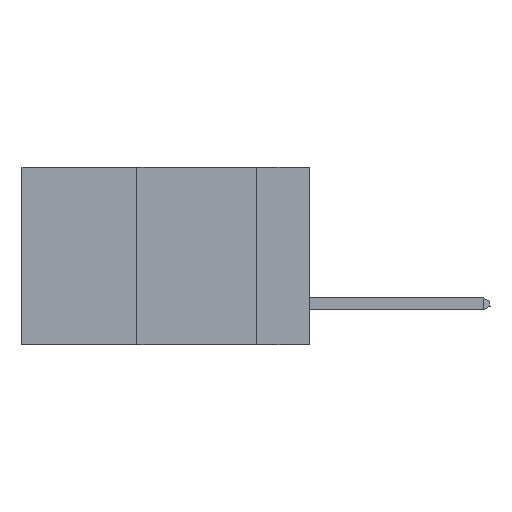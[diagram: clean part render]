
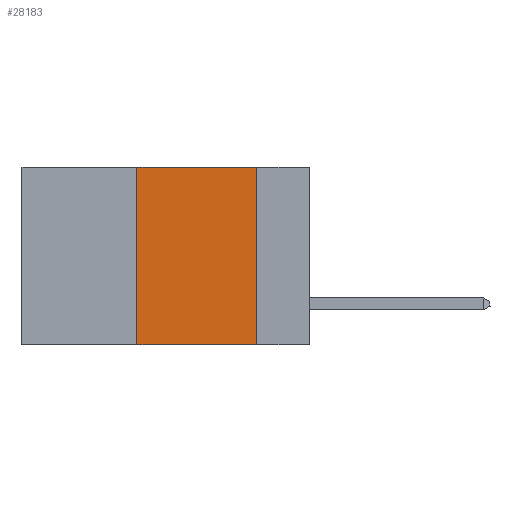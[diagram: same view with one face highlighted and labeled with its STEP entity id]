
A CAD part, left-side view. The second image highlights one B-rep face of the part: STEP entity #28183.
In plain terms, the highlighted planar face has unit normal (-1, 0, 0).
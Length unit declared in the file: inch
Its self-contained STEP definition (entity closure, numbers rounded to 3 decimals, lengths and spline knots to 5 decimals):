
#24 = CARTESIAN_POINT ( 'NONE',  ( 0., 0.36, 0. ) ) ;
#394 = CARTESIAN_POINT ( 'NONE',  ( 0., 0.36, 0. ) ) ;
#823 = LINE ( 'NONE', #1467, #23606 ) ;
#988 = VECTOR ( 'NONE', #38462, 39.37008 ) ;
#1054 = ORIENTED_EDGE ( 'NONE', *, *, #20880, .F. ) ;
#1467 = CARTESIAN_POINT ( 'NONE',  ( 0., 0.6, 0. ) ) ;
#1774 = CARTESIAN_POINT ( 'NONE',  ( 0., 0.11, 0. ) ) ;
#3610 = DIRECTION ( 'NONE',  ( 1., 0., 0. ) ) ;
#4668 = ORIENTED_EDGE ( 'NONE', *, *, #29044, .T. ) ;
#6092 = CARTESIAN_POINT ( 'NONE',  ( 0., 0.6, 0. ) ) ;
#6477 = DIRECTION ( 'NONE',  ( 0., 0., -1. ) ) ;
#12211 = ORIENTED_EDGE ( 'NONE', *, *, #37625, .F. ) ;
#16235 = DIRECTION ( 'NONE',  ( 0., -1., 0. ) ) ;
#16860 = FACE_OUTER_BOUND ( 'NONE', #23038, .T. ) ;
#17054 = VERTEX_POINT ( 'NONE', #27742 ) ;
#19706 = LINE ( 'NONE', #394, #21110 ) ;
#20880 = EDGE_CURVE ( 'NONE', #34108, #36060, #823, .T. ) ;
#21110 = VECTOR ( 'NONE', #24189, 39.37008 ) ;
#21430 = LINE ( 'NONE', #38340, #988 ) ;
#23038 = EDGE_LOOP ( 'NONE', ( #12211, #1054, #27470, #4668 ) ) ;
#23311 = LINE ( 'NONE', #30259, #37299 ) ;
#23606 = VECTOR ( 'NONE', #16235, 39.37008 ) ;
#24189 = DIRECTION ( 'NONE',  ( 0., 0., 1. ) ) ;
#24332 = CARTESIAN_POINT ( 'NONE',  ( 0., 0.11, -0.37 ) ) ;
#24414 = AXIS2_PLACEMENT_3D ( 'NONE', #6092, #3610, #6477 ) ;
#27415 = DIRECTION ( 'NONE',  ( 0., -1., 0. ) ) ;
#27470 = ORIENTED_EDGE ( 'NONE', *, *, #27491, .F. ) ;
#27491 = EDGE_CURVE ( 'NONE', #17054, #34108, #19706, .T. ) ;
#27742 = CARTESIAN_POINT ( 'NONE',  ( 0., 0.36, -0.37 ) ) ;
#28183 = ADVANCED_FACE ( 'NONE', ( #16860 ), #32981, .F. ) ;
#28251 = VERTEX_POINT ( 'NONE', #24332 ) ;
#29044 = EDGE_CURVE ( 'NONE', #17054, #28251, #23311, .T. ) ;
#30259 = CARTESIAN_POINT ( 'NONE',  ( 0., 0.6, -0.37 ) ) ;
#32981 = PLANE ( 'NONE',  #24414 ) ;
#34108 = VERTEX_POINT ( 'NONE', #24 ) ;
#36060 = VERTEX_POINT ( 'NONE', #1774 ) ;
#37299 = VECTOR ( 'NONE', #27415, 39.37008 ) ;
#37625 = EDGE_CURVE ( 'NONE', #36060, #28251, #21430, .T. ) ;
#38340 = CARTESIAN_POINT ( 'NONE',  ( 0., 0.11, 0. ) ) ;
#38462 = DIRECTION ( 'NONE',  ( 0., 0., -1. ) ) ;
